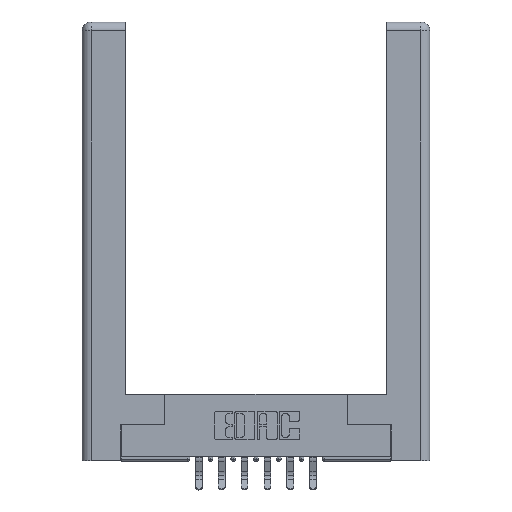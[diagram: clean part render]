
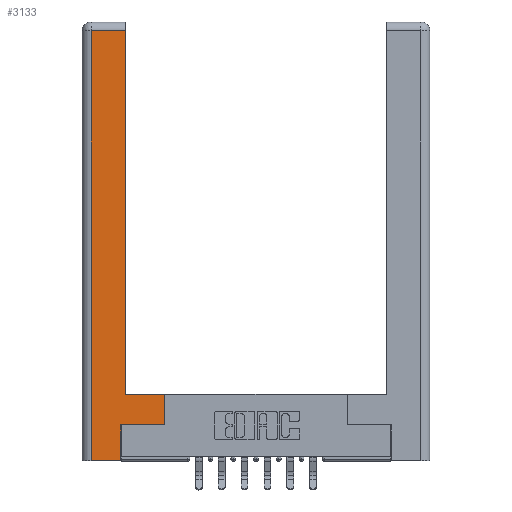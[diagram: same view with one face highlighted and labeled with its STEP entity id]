
A CAD part, top view. The second image highlights one B-rep face of the part: STEP entity #3133.
In plain terms, the highlighted planar face has unit normal (0, 0, 1).
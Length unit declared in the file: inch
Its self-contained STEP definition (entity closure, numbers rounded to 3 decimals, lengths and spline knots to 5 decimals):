
#50 = VERTEX_POINT ( 'NONE', #13317 ) ;
#72 = DIRECTION ( 'NONE',  ( 0., 1., 0. ) ) ;
#757 = DIRECTION ( 'NONE',  ( 0., 1., 0. ) ) ;
#790 = CARTESIAN_POINT ( 'NONE',  ( 0.0615, 0., 0. ) ) ;
#933 = EDGE_CURVE ( 'NONE', #11781, #10602, #8794, .T. ) ;
#947 = VECTOR ( 'NONE', #11472, 39.37008 ) ;
#1211 = ORIENTED_EDGE ( 'NONE', *, *, #933, .T. ) ;
#1225 = DIRECTION ( 'NONE',  ( 1., 0., 0. ) ) ;
#1241 = DIRECTION ( 'NONE',  ( -1., 0., 0. ) ) ;
#2084 = CARTESIAN_POINT ( 'NONE',  ( 0.265, 0., 0. ) ) ;
#2117 = ORIENTED_EDGE ( 'NONE', *, *, #11114, .T. ) ;
#2138 = CARTESIAN_POINT ( 'NONE',  ( 0.295, 2.94, 0. ) ) ;
#2218 = VECTOR ( 'NONE', #72, 39.37008 ) ;
#2350 = CARTESIAN_POINT ( 'NONE',  ( 0.0615, 2.94, 0. ) ) ;
#2453 = FACE_OUTER_BOUND ( 'NONE', #12298, .T. ) ;
#2518 = EDGE_CURVE ( 'NONE', #10040, #12264, #12438, .T. ) ;
#2725 = CARTESIAN_POINT ( 'NONE',  ( 0.295, 3., 0. ) ) ;
#3133 = ADVANCED_FACE ( 'NONE', ( #2453 ), #3532, .F. ) ;
#3213 = CARTESIAN_POINT ( 'NONE',  ( 0.295, 0.45, 0. ) ) ;
#3230 = VERTEX_POINT ( 'NONE', #8214 ) ;
#3465 = DIRECTION ( 'NONE',  ( -1., 0., 0. ) ) ;
#3532 = PLANE ( 'NONE',  #10308 ) ;
#3861 = ORIENTED_EDGE ( 'NONE', *, *, #12738, .T. ) ;
#3986 = VECTOR ( 'NONE', #3465, 39.37008 ) ;
#4064 = ORIENTED_EDGE ( 'NONE', *, *, #13244, .T. ) ;
#4250 = LINE ( 'NONE', #9673, #2218 ) ;
#4260 = ORIENTED_EDGE ( 'NONE', *, *, #10498, .T. ) ;
#4922 = DIRECTION ( 'NONE',  ( 0., -1., 0. ) ) ;
#5227 = EDGE_CURVE ( 'NONE', #13170, #10040, #4250, .T. ) ;
#5317 = CARTESIAN_POINT ( 'NONE',  ( 0.565, 0.45, 0. ) ) ;
#5325 = DIRECTION ( 'NONE',  ( 1., 0., 0. ) ) ;
#5475 = CARTESIAN_POINT ( 'NONE',  ( 0., 0., 0. ) ) ;
#5660 = VECTOR ( 'NONE', #11734, 39.37008 ) ;
#6022 = CARTESIAN_POINT ( 'NONE',  ( 0.565, 0.45, 0. ) ) ;
#6115 = CARTESIAN_POINT ( 'NONE',  ( 0.565, 0.245, 0. ) ) ;
#6256 = LINE ( 'NONE', #2725, #12680 ) ;
#6535 = DIRECTION ( 'NONE',  ( 0., 0., -1. ) ) ;
#6619 = ORIENTED_EDGE ( 'NONE', *, *, #5227, .T. ) ;
#6973 = CARTESIAN_POINT ( 'NONE',  ( 0.265, 0., 0. ) ) ;
#7463 = LINE ( 'NONE', #2084, #7975 ) ;
#7465 = VECTOR ( 'NONE', #5325, 39.37008 ) ;
#7975 = VECTOR ( 'NONE', #1225, 39.37008 ) ;
#7982 = CARTESIAN_POINT ( 'NONE',  ( 0.265, 0.245, 0. ) ) ;
#8214 = CARTESIAN_POINT ( 'NONE',  ( 0.0615, 0., 0. ) ) ;
#8794 = LINE ( 'NONE', #11562, #947 ) ;
#8801 = LINE ( 'NONE', #5317, #5660 ) ;
#9673 = CARTESIAN_POINT ( 'NONE',  ( 0.265, 0.245, 0. ) ) ;
#10040 = VERTEX_POINT ( 'NONE', #7982 ) ;
#10308 = AXIS2_PLACEMENT_3D ( 'NONE', #5475, #6535, #1241 ) ;
#10449 = EDGE_CURVE ( 'NONE', #3230, #13170, #7463, .T. ) ;
#10498 = EDGE_CURVE ( 'NONE', #12264, #11781, #8801, .T. ) ;
#10602 = VERTEX_POINT ( 'NONE', #3213 ) ;
#11114 = EDGE_CURVE ( 'NONE', #13314, #50, #12893, .T. ) ;
#11200 = LINE ( 'NONE', #790, #12669 ) ;
#11472 = DIRECTION ( 'NONE',  ( -1., 0., 0. ) ) ;
#11562 = CARTESIAN_POINT ( 'NONE',  ( 0.295, 0.45, 0. ) ) ;
#11661 = CARTESIAN_POINT ( 'NONE',  ( 0.565, 0.245, 0. ) ) ;
#11734 = DIRECTION ( 'NONE',  ( 0., 1., 0. ) ) ;
#11781 = VERTEX_POINT ( 'NONE', #6022 ) ;
#12196 = ORIENTED_EDGE ( 'NONE', *, *, #10449, .T. ) ;
#12264 = VERTEX_POINT ( 'NONE', #6115 ) ;
#12298 = EDGE_LOOP ( 'NONE', ( #3861, #2117, #4064, #12196, #6619, #12759, #4260, #1211 ) ) ;
#12438 = LINE ( 'NONE', #11661, #7465 ) ;
#12669 = VECTOR ( 'NONE', #4922, 39.37008 ) ;
#12680 = VECTOR ( 'NONE', #757, 39.37008 ) ;
#12738 = EDGE_CURVE ( 'NONE', #10602, #13314, #6256, .T. ) ;
#12759 = ORIENTED_EDGE ( 'NONE', *, *, #2518, .T. ) ;
#12893 = LINE ( 'NONE', #2350, #3986 ) ;
#13170 = VERTEX_POINT ( 'NONE', #6973 ) ;
#13244 = EDGE_CURVE ( 'NONE', #50, #3230, #11200, .T. ) ;
#13314 = VERTEX_POINT ( 'NONE', #2138 ) ;
#13317 = CARTESIAN_POINT ( 'NONE',  ( 0.0615, 2.94, 0. ) ) ;
